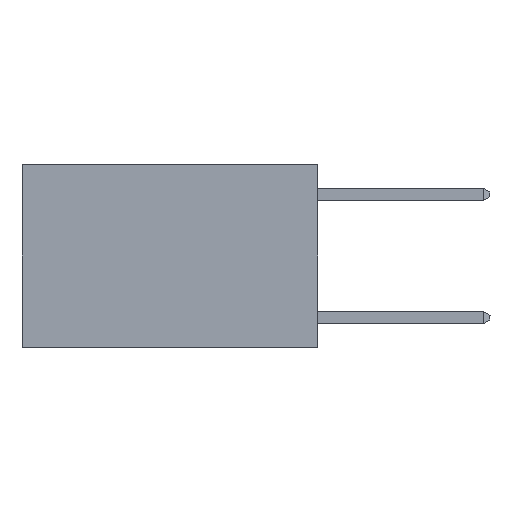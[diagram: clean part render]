
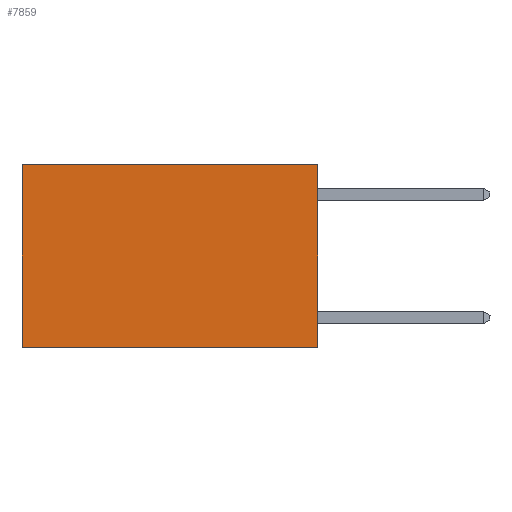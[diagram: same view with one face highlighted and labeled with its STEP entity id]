
A CAD part, left-side view. The second image highlights one B-rep face of the part: STEP entity #7859.
In plain terms, the highlighted planar face has unit normal (-1, 0, 0).
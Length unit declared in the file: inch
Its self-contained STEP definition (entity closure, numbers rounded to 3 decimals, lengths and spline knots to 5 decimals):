
#9 = VERTEX_POINT ( 'NONE', #3023 ) ;
#316 = EDGE_LOOP ( 'NONE', ( #7339, #3611, #7758, #1116 ) ) ;
#396 = VERTEX_POINT ( 'NONE', #10149 ) ;
#441 = DIRECTION ( 'NONE',  ( 0., 1., 0. ) ) ;
#649 = CARTESIAN_POINT ( 'NONE',  ( 0.2625, 0., 0. ) ) ;
#919 = LINE ( 'NONE', #1249, #9770 ) ;
#928 = FACE_OUTER_BOUND ( 'NONE', #316, .T. ) ;
#1006 = DIRECTION ( 'NONE',  ( 0., 1., 0. ) ) ;
#1116 = ORIENTED_EDGE ( 'NONE', *, *, #9007, .T. ) ;
#1249 = CARTESIAN_POINT ( 'NONE',  ( 0.2625, 0., -0.37 ) ) ;
#1422 = LINE ( 'NONE', #3791, #10274 ) ;
#1427 = EDGE_CURVE ( 'NONE', #9, #1701, #919, .T. ) ;
#1559 = EDGE_CURVE ( 'NONE', #396, #1701, #8538, .T. ) ;
#1701 = VERTEX_POINT ( 'NONE', #4770 ) ;
#2118 = DIRECTION ( 'NONE',  ( 0., 0., -1. ) ) ;
#2122 = LINE ( 'NONE', #7873, #10948 ) ;
#2978 = DIRECTION ( 'NONE',  ( 1., 0., 0. ) ) ;
#3023 = CARTESIAN_POINT ( 'NONE',  ( 0.2625, 0., -0.37 ) ) ;
#3125 = DIRECTION ( 'NONE',  ( 0., 0., -1. ) ) ;
#3499 = EDGE_CURVE ( 'NONE', #3950, #9, #1422, .T. ) ;
#3611 = ORIENTED_EDGE ( 'NONE', *, *, #1427, .F. ) ;
#3791 = CARTESIAN_POINT ( 'NONE',  ( 0.2625, 0., 0. ) ) ;
#3950 = VERTEX_POINT ( 'NONE', #649 ) ;
#4735 = CARTESIAN_POINT ( 'NONE',  ( 0.2625, 0., 0. ) ) ;
#4770 = CARTESIAN_POINT ( 'NONE',  ( 0.2625, 0.6, -0.37 ) ) ;
#4933 = VECTOR ( 'NONE', #3125, 39.37008 ) ;
#5687 = CARTESIAN_POINT ( 'NONE',  ( 0.2625, 0.6, 0. ) ) ;
#7195 = PLANE ( 'NONE',  #7847 ) ;
#7339 = ORIENTED_EDGE ( 'NONE', *, *, #1559, .T. ) ;
#7758 = ORIENTED_EDGE ( 'NONE', *, *, #3499, .F. ) ;
#7847 = AXIS2_PLACEMENT_3D ( 'NONE', #4735, #2978, #8958 ) ;
#7859 = ADVANCED_FACE ( 'NONE', ( #928 ), #7195, .F. ) ;
#7873 = CARTESIAN_POINT ( 'NONE',  ( 0.2625, 0., 0. ) ) ;
#8538 = LINE ( 'NONE', #5687, #4933 ) ;
#8958 = DIRECTION ( 'NONE',  ( 0., 0., -1. ) ) ;
#9007 = EDGE_CURVE ( 'NONE', #3950, #396, #2122, .T. ) ;
#9770 = VECTOR ( 'NONE', #441, 39.37008 ) ;
#10149 = CARTESIAN_POINT ( 'NONE',  ( 0.2625, 0.6, 0. ) ) ;
#10274 = VECTOR ( 'NONE', #2118, 39.37008 ) ;
#10948 = VECTOR ( 'NONE', #1006, 39.37008 ) ;
